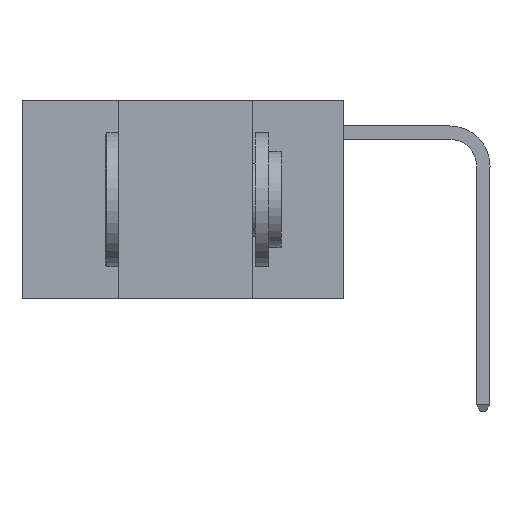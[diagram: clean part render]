
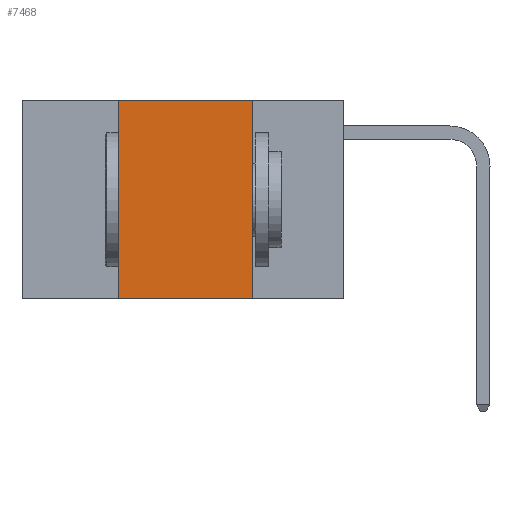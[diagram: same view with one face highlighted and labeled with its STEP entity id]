
A CAD part, left-side view. The second image highlights one B-rep face of the part: STEP entity #7468.
In plain terms, the highlighted planar face has unit normal (-1, 0, 0).
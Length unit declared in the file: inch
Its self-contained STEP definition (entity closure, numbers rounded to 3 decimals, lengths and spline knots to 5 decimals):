
#539 = DIRECTION ( 'NONE',  ( 0., -1., 0. ) ) ;
#744 = DIRECTION ( 'NONE',  ( 0., 0., 1. ) ) ;
#817 = CARTESIAN_POINT ( 'NONE',  ( 0., 0.42, -0.37 ) ) ;
#1155 = FACE_OUTER_BOUND ( 'NONE', #6634, .T. ) ;
#1313 = VECTOR ( 'NONE', #539, 39.37008 ) ;
#2044 = LINE ( 'NONE', #14224, #1313 ) ;
#2084 = EDGE_CURVE ( 'NONE', #12715, #12390, #14160, .T. ) ;
#2580 = EDGE_CURVE ( 'NONE', #12715, #9359, #7772, .T. ) ;
#2808 = ORIENTED_EDGE ( 'NONE', *, *, #2580, .T. ) ;
#3818 = DIRECTION ( 'NONE',  ( 0., -1., 0. ) ) ;
#4099 = PLANE ( 'NONE',  #6487 ) ;
#4170 = CARTESIAN_POINT ( 'NONE',  ( 0., 0.42, 0. ) ) ;
#5570 = VERTEX_POINT ( 'NONE', #6272 ) ;
#6272 = CARTESIAN_POINT ( 'NONE',  ( 0., 0.17, 0. ) ) ;
#6382 = CARTESIAN_POINT ( 'NONE',  ( 0., 0.6, 0. ) ) ;
#6487 = AXIS2_PLACEMENT_3D ( 'NONE', #6382, #14336, #7576 ) ;
#6634 = EDGE_LOOP ( 'NONE', ( #10855, #11209, #14203, #2808 ) ) ;
#6745 = LINE ( 'NONE', #12062, #12480 ) ;
#6810 = EDGE_CURVE ( 'NONE', #5570, #9359, #6745, .T. ) ;
#7468 = ADVANCED_FACE ( 'NONE', ( #1155 ), #4099, .F. ) ;
#7576 = DIRECTION ( 'NONE',  ( 0., 0., -1. ) ) ;
#7772 = LINE ( 'NONE', #8419, #8112 ) ;
#8112 = VECTOR ( 'NONE', #3818, 39.37008 ) ;
#8419 = CARTESIAN_POINT ( 'NONE',  ( 0., 0.6, -0.37 ) ) ;
#8614 = EDGE_CURVE ( 'NONE', #12390, #5570, #2044, .T. ) ;
#9359 = VERTEX_POINT ( 'NONE', #14340 ) ;
#10855 = ORIENTED_EDGE ( 'NONE', *, *, #6810, .F. ) ;
#10908 = DIRECTION ( 'NONE',  ( 0., 0., -1. ) ) ;
#11159 = VECTOR ( 'NONE', #744, 39.37008 ) ;
#11209 = ORIENTED_EDGE ( 'NONE', *, *, #8614, .F. ) ;
#11779 = CARTESIAN_POINT ( 'NONE',  ( 0., 0.42, 0. ) ) ;
#12062 = CARTESIAN_POINT ( 'NONE',  ( 0., 0.17, 0. ) ) ;
#12390 = VERTEX_POINT ( 'NONE', #11779 ) ;
#12480 = VECTOR ( 'NONE', #10908, 39.37008 ) ;
#12715 = VERTEX_POINT ( 'NONE', #817 ) ;
#14160 = LINE ( 'NONE', #4170, #11159 ) ;
#14203 = ORIENTED_EDGE ( 'NONE', *, *, #2084, .F. ) ;
#14224 = CARTESIAN_POINT ( 'NONE',  ( 0., 0.6, 0. ) ) ;
#14336 = DIRECTION ( 'NONE',  ( 1., 0., 0. ) ) ;
#14340 = CARTESIAN_POINT ( 'NONE',  ( 0., 0.17, -0.37 ) ) ;
